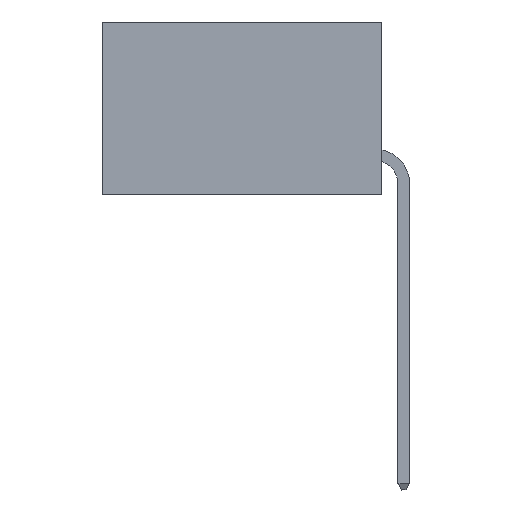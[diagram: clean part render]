
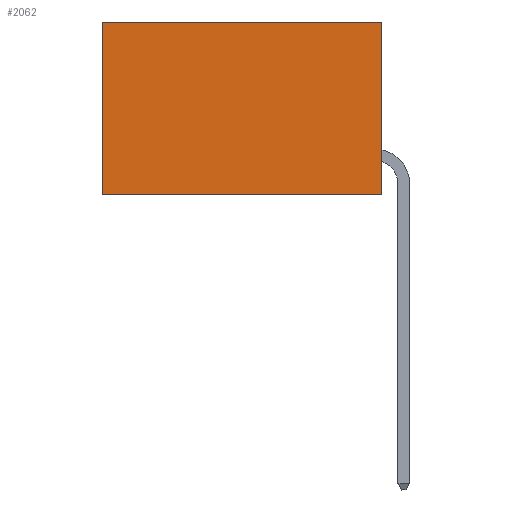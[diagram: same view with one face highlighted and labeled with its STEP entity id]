
A CAD part, left-side view. The second image highlights one B-rep face of the part: STEP entity #2062.
In plain terms, the highlighted planar face has unit normal (-1, 0, 0).
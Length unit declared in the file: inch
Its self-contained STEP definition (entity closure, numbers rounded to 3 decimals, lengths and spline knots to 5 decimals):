
#751 = EDGE_LOOP ( 'NONE', ( #12216, #35107, #27984, #39616 ) ) ;
#1533 = CARTESIAN_POINT ( 'NONE',  ( 0.2875, 0., -0.37 ) ) ;
#1951 = DIRECTION ( 'NONE',  ( 0., 1., 0. ) ) ;
#2062 = ADVANCED_FACE ( 'NONE', ( #3332 ), #15039, .F. ) ;
#2213 = LINE ( 'NONE', #31746, #27806 ) ;
#3332 = FACE_OUTER_BOUND ( 'NONE', #751, .T. ) ;
#3581 = LINE ( 'NONE', #1533, #20989 ) ;
#4399 = CARTESIAN_POINT ( 'NONE',  ( 0.2875, 0.6, -0.37 ) ) ;
#4627 = VECTOR ( 'NONE', #13572, 39.37008 ) ;
#4925 = CARTESIAN_POINT ( 'NONE',  ( 0.2875, 0., 0. ) ) ;
#5167 = DIRECTION ( 'NONE',  ( 0., 0., -1. ) ) ;
#6079 = CARTESIAN_POINT ( 'NONE',  ( 0.2875, 0., 0. ) ) ;
#9782 = CARTESIAN_POINT ( 'NONE',  ( 0.2875, 0., 0. ) ) ;
#10917 = LINE ( 'NONE', #9782, #4627 ) ;
#10982 = VERTEX_POINT ( 'NONE', #27088 ) ;
#12216 = ORIENTED_EDGE ( 'NONE', *, *, #32797, .T. ) ;
#13572 = DIRECTION ( 'NONE',  ( 0., 1., 0. ) ) ;
#14179 = VERTEX_POINT ( 'NONE', #4925 ) ;
#14213 = EDGE_CURVE ( 'NONE', #14179, #10982, #10917, .T. ) ;
#14906 = DIRECTION ( 'NONE',  ( 0., 0., -1. ) ) ;
#15039 = PLANE ( 'NONE',  #32444 ) ;
#19018 = LINE ( 'NONE', #23251, #24277 ) ;
#20989 = VECTOR ( 'NONE', #1951, 39.37008 ) ;
#22928 = DIRECTION ( 'NONE',  ( 0., 0., -1. ) ) ;
#23251 = CARTESIAN_POINT ( 'NONE',  ( 0.2875, 0., 0. ) ) ;
#24277 = VECTOR ( 'NONE', #5167, 39.37008 ) ;
#25813 = CARTESIAN_POINT ( 'NONE',  ( 0.2875, 0., -0.37 ) ) ;
#27088 = CARTESIAN_POINT ( 'NONE',  ( 0.2875, 0.6, 0. ) ) ;
#27579 = VERTEX_POINT ( 'NONE', #4399 ) ;
#27806 = VECTOR ( 'NONE', #22928, 39.37008 ) ;
#27984 = ORIENTED_EDGE ( 'NONE', *, *, #39973, .F. ) ;
#31746 = CARTESIAN_POINT ( 'NONE',  ( 0.2875, 0.6, 0. ) ) ;
#32444 = AXIS2_PLACEMENT_3D ( 'NONE', #6079, #39828, #14906 ) ;
#32797 = EDGE_CURVE ( 'NONE', #10982, #27579, #2213, .T. ) ;
#35107 = ORIENTED_EDGE ( 'NONE', *, *, #39228, .F. ) ;
#39228 = EDGE_CURVE ( 'NONE', #39850, #27579, #3581, .T. ) ;
#39616 = ORIENTED_EDGE ( 'NONE', *, *, #14213, .T. ) ;
#39828 = DIRECTION ( 'NONE',  ( 1., 0., 0. ) ) ;
#39850 = VERTEX_POINT ( 'NONE', #25813 ) ;
#39973 = EDGE_CURVE ( 'NONE', #14179, #39850, #19018, .T. ) ;
